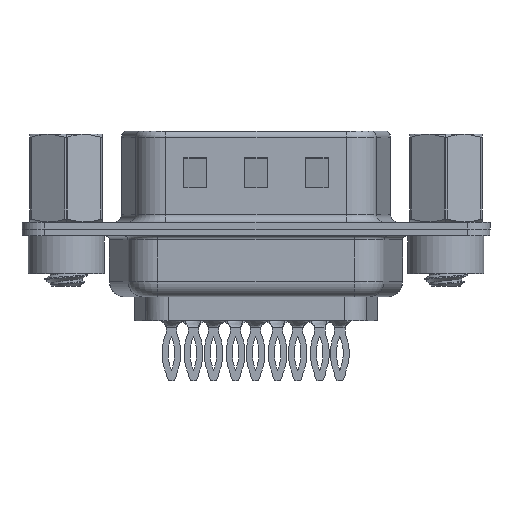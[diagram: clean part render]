
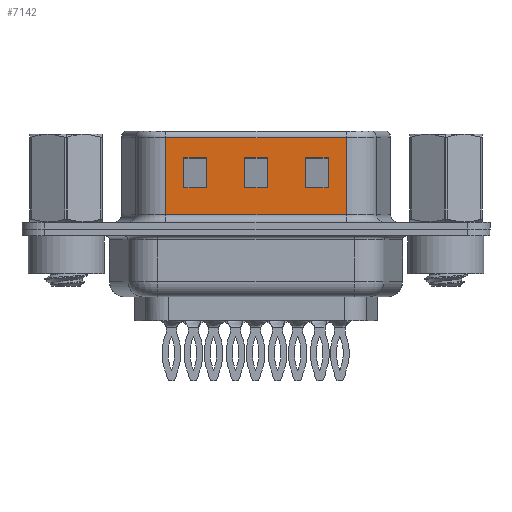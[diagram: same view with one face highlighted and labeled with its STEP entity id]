
A CAD part, front view. The second image highlights one B-rep face of the part: STEP entity #7142.
In plain terms, the highlighted planar face has unit normal (0, -1, 0).
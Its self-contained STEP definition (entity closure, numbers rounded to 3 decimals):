
#5 = CARTESIAN_POINT ( 'NONE',  ( 22.445, -4.58, 2.705 ) ) ;
#225 = LINE ( 'NONE', #5, #17846 ) ;
#281 = AXIS2_PLACEMENT_3D ( 'NONE', #5912, #15935, #12637 ) ;
#364 = LINE ( 'NONE', #13672, #9409 ) ;
#991 = VECTOR ( 'NONE', #17453, 1000. ) ;
#1026 = VECTOR ( 'NONE', #21370, 1000. ) ;
#1065 = VERTEX_POINT ( 'NONE', #5603 ) ;
#1172 = ORIENTED_EDGE ( 'NONE', *, *, #15927, .T. ) ;
#1427 = VECTOR ( 'NONE', #1695, 1000. ) ;
#1654 = CARTESIAN_POINT ( 'NONE',  ( 17.245, -4.58, 2.705 ) ) ;
#1695 = DIRECTION ( 'NONE',  ( 0., 0., -1. ) ) ;
#1793 = CARTESIAN_POINT ( 'NONE',  ( 18.445, -4.58, 6.02 ) ) ;
#1898 = DIRECTION ( 'NONE',  ( -1., 0., 0. ) ) ;
#2000 = CARTESIAN_POINT ( 'NONE',  ( 7.745, -4.58, 6.52 ) ) ;
#2476 = VERTEX_POINT ( 'NONE', #20648 ) ;
#2485 = LINE ( 'NONE', #5687, #7076 ) ;
#2727 = FACE_BOUND ( 'NONE', #14940, .T. ) ;
#2777 = LINE ( 'NONE', #15978, #19882 ) ;
#2922 = LINE ( 'NONE', #4166, #14982 ) ;
#3330 = EDGE_LOOP ( 'NONE', ( #14161, #1172, #11680, #15747 ) ) ;
#3653 = ORIENTED_EDGE ( 'NONE', *, *, #10242, .T. ) ;
#3658 = ORIENTED_EDGE ( 'NONE', *, *, #15259, .T. ) ;
#3674 = EDGE_CURVE ( 'NONE', #1065, #19030, #15326, .T. ) ;
#3750 = CARTESIAN_POINT ( 'NONE',  ( 18.445, -4.58, 0.95 ) ) ;
#3858 = EDGE_CURVE ( 'NONE', #8471, #17684, #20876, .T. ) ;
#4065 = VERTEX_POINT ( 'NONE', #12612 ) ;
#4166 = CARTESIAN_POINT ( 'NONE',  ( 18.445, -4.58, 6.52 ) ) ;
#4791 = CARTESIAN_POINT ( 'NONE',  ( 7.745, -4.58, 4.705 ) ) ;
#5521 = LINE ( 'NONE', #8393, #10117 ) ;
#5603 = CARTESIAN_POINT ( 'NONE',  ( 18.445, -4.58, 6.02 ) ) ;
#5687 = CARTESIAN_POINT ( 'NONE',  ( 9.245, -4.58, 6.52 ) ) ;
#5754 = CARTESIAN_POINT ( 'NONE',  ( 11.745, -4.58, 6.52 ) ) ;
#5912 = CARTESIAN_POINT ( 'NONE',  ( 18.445, -4.58, 6.52 ) ) ;
#5944 = ORIENTED_EDGE ( 'NONE', *, *, #3858, .T. ) ;
#6185 = CARTESIAN_POINT ( 'NONE',  ( 6.545, -4.58, 6.02 ) ) ;
#6193 = VERTEX_POINT ( 'NONE', #7801 ) ;
#6239 = FACE_OUTER_BOUND ( 'NONE', #19968, .T. ) ;
#6380 = VECTOR ( 'NONE', #11335, 1000. ) ;
#6663 = CARTESIAN_POINT ( 'NONE',  ( 17.245, -4.58, 4.705 ) ) ;
#6908 = EDGE_CURVE ( 'NONE', #2476, #15737, #14059, .T. ) ;
#7076 = VECTOR ( 'NONE', #19087, 1000. ) ;
#7142 = ADVANCED_FACE ( 'NONE', ( #17566, #2727, #9434, #6239 ), #11308, .F. ) ;
#7801 = CARTESIAN_POINT ( 'NONE',  ( 11.745, -4.58, 4.705 ) ) ;
#8067 = LINE ( 'NONE', #14779, #1026 ) ;
#8137 = ORIENTED_EDGE ( 'NONE', *, *, #3674, .T. ) ;
#8382 = LINE ( 'NONE', #10254, #10697 ) ;
#8393 = CARTESIAN_POINT ( 'NONE',  ( 15.745, -4.58, 6.52 ) ) ;
#8471 = VERTEX_POINT ( 'NONE', #14948 ) ;
#8583 = EDGE_CURVE ( 'NONE', #18231, #8471, #2485, .T. ) ;
#8639 = LINE ( 'NONE', #15351, #14020 ) ;
#8955 = VERTEX_POINT ( 'NONE', #4791 ) ;
#9123 = DIRECTION ( 'NONE',  ( 1., 0., 0. ) ) ;
#9203 = EDGE_LOOP ( 'NONE', ( #13097, #5944, #3658, #3653 ) ) ;
#9338 = ORIENTED_EDGE ( 'NONE', *, *, #15983, .T. ) ;
#9409 = VECTOR ( 'NONE', #16849, 1000. ) ;
#9434 = FACE_BOUND ( 'NONE', #3330, .T. ) ;
#9868 = ORIENTED_EDGE ( 'NONE', *, *, #12613, .T. ) ;
#9917 = VERTEX_POINT ( 'NONE', #21143 ) ;
#9960 = LINE ( 'NONE', #21500, #1427 ) ;
#10117 = VECTOR ( 'NONE', #18385, 1000. ) ;
#10242 = EDGE_CURVE ( 'NONE', #8955, #18231, #8382, .T. ) ;
#10254 = CARTESIAN_POINT ( 'NONE',  ( 14.445, -4.58, 4.705 ) ) ;
#10598 = LINE ( 'NONE', #2000, #15352 ) ;
#10697 = VECTOR ( 'NONE', #9123, 1000. ) ;
#11041 = CARTESIAN_POINT ( 'NONE',  ( 7.745, -4.58, 2.705 ) ) ;
#11055 = EDGE_CURVE ( 'NONE', #19030, #9917, #9960, .T. ) ;
#11245 = DIRECTION ( 'NONE',  ( 0., 0., -1. ) ) ;
#11308 = PLANE ( 'NONE',  #281 ) ;
#11335 = DIRECTION ( 'NONE',  ( -1., 0., 0. ) ) ;
#11680 = ORIENTED_EDGE ( 'NONE', *, *, #6908, .T. ) ;
#12158 = DIRECTION ( 'NONE',  ( 1., 0., 0. ) ) ;
#12289 = EDGE_CURVE ( 'NONE', #6193, #4065, #21260, .T. ) ;
#12291 = CARTESIAN_POINT ( 'NONE',  ( 15.745, -4.58, 2.705 ) ) ;
#12474 = DIRECTION ( 'NONE',  ( 0., 0., 1. ) ) ;
#12612 = CARTESIAN_POINT ( 'NONE',  ( 13.245, -4.58, 4.705 ) ) ;
#12613 = EDGE_CURVE ( 'NONE', #13253, #15501, #2777, .T. ) ;
#12637 = DIRECTION ( 'NONE',  ( 0., 0., 1. ) ) ;
#12755 = ORIENTED_EDGE ( 'NONE', *, *, #14931, .F. ) ;
#13097 = ORIENTED_EDGE ( 'NONE', *, *, #8583, .T. ) ;
#13253 = VERTEX_POINT ( 'NONE', #6663 ) ;
#13589 = VECTOR ( 'NONE', #16004, 1000. ) ;
#13672 = CARTESIAN_POINT ( 'NONE',  ( 13.245, -4.58, 6.52 ) ) ;
#14020 = VECTOR ( 'NONE', #12158, 1000. ) ;
#14059 = LINE ( 'NONE', #17239, #991 ) ;
#14118 = LINE ( 'NONE', #5754, #15498 ) ;
#14161 = ORIENTED_EDGE ( 'NONE', *, *, #12289, .T. ) ;
#14221 = DIRECTION ( 'NONE',  ( 0., 0., 1. ) ) ;
#14258 = VERTEX_POINT ( 'NONE', #3750 ) ;
#14417 = ORIENTED_EDGE ( 'NONE', *, *, #17082, .T. ) ;
#14779 = CARTESIAN_POINT ( 'NONE',  ( 22.445, -4.58, 4.705 ) ) ;
#14931 = EDGE_CURVE ( 'NONE', #1065, #14258, #2922, .T. ) ;
#14940 = EDGE_LOOP ( 'NONE', ( #9868, #21026, #9338, #17110 ) ) ;
#14948 = CARTESIAN_POINT ( 'NONE',  ( 9.245, -4.58, 2.705 ) ) ;
#14982 = VECTOR ( 'NONE', #21485, 1000. ) ;
#15259 = EDGE_CURVE ( 'NONE', #17684, #8955, #10598, .T. ) ;
#15326 = LINE ( 'NONE', #1793, #20735 ) ;
#15351 = CARTESIAN_POINT ( 'NONE',  ( 18.445, -4.58, 0.95 ) ) ;
#15352 = VECTOR ( 'NONE', #14221, 1000. ) ;
#15498 = VECTOR ( 'NONE', #12474, 1000. ) ;
#15501 = VERTEX_POINT ( 'NONE', #1654 ) ;
#15583 = ORIENTED_EDGE ( 'NONE', *, *, #11055, .T. ) ;
#15737 = VERTEX_POINT ( 'NONE', #17444 ) ;
#15747 = ORIENTED_EDGE ( 'NONE', *, *, #19170, .T. ) ;
#15892 = VERTEX_POINT ( 'NONE', #12291 ) ;
#15927 = EDGE_CURVE ( 'NONE', #4065, #2476, #364, .T. ) ;
#15935 = DIRECTION ( 'NONE',  ( 0., 1., 0. ) ) ;
#15978 = CARTESIAN_POINT ( 'NONE',  ( 17.245, -4.58, 6.52 ) ) ;
#15983 = EDGE_CURVE ( 'NONE', #15892, #17719, #5521, .T. ) ;
#16004 = DIRECTION ( 'NONE',  ( 1., 0., 0. ) ) ;
#16308 = EDGE_CURVE ( 'NONE', #15501, #15892, #225, .T. ) ;
#16821 = DIRECTION ( 'NONE',  ( -1., 0., 0. ) ) ;
#16849 = DIRECTION ( 'NONE',  ( 0., 0., -1. ) ) ;
#17082 = EDGE_CURVE ( 'NONE', #9917, #14258, #8639, .T. ) ;
#17110 = ORIENTED_EDGE ( 'NONE', *, *, #17312, .T. ) ;
#17239 = CARTESIAN_POINT ( 'NONE',  ( 18.445, -4.58, 2.705 ) ) ;
#17312 = EDGE_CURVE ( 'NONE', #17719, #13253, #8067, .T. ) ;
#17444 = CARTESIAN_POINT ( 'NONE',  ( 11.745, -4.58, 2.705 ) ) ;
#17453 = DIRECTION ( 'NONE',  ( -1., 0., 0. ) ) ;
#17566 = FACE_BOUND ( 'NONE', #9203, .T. ) ;
#17646 = CARTESIAN_POINT ( 'NONE',  ( 18.445, -4.58, 4.705 ) ) ;
#17684 = VERTEX_POINT ( 'NONE', #11041 ) ;
#17719 = VERTEX_POINT ( 'NONE', #17946 ) ;
#17846 = VECTOR ( 'NONE', #16821, 1000. ) ;
#17946 = CARTESIAN_POINT ( 'NONE',  ( 15.745, -4.58, 4.705 ) ) ;
#18119 = CARTESIAN_POINT ( 'NONE',  ( 9.245, -4.58, 4.705 ) ) ;
#18231 = VERTEX_POINT ( 'NONE', #18119 ) ;
#18385 = DIRECTION ( 'NONE',  ( 0., 0., 1. ) ) ;
#19030 = VERTEX_POINT ( 'NONE', #6185 ) ;
#19087 = DIRECTION ( 'NONE',  ( 0., 0., -1. ) ) ;
#19170 = EDGE_CURVE ( 'NONE', #15737, #6193, #14118, .T. ) ;
#19236 = CARTESIAN_POINT ( 'NONE',  ( 14.445, -4.58, 2.705 ) ) ;
#19882 = VECTOR ( 'NONE', #11245, 1000. ) ;
#19968 = EDGE_LOOP ( 'NONE', ( #12755, #8137, #15583, #14417 ) ) ;
#20648 = CARTESIAN_POINT ( 'NONE',  ( 13.245, -4.58, 2.705 ) ) ;
#20735 = VECTOR ( 'NONE', #1898, 1000. ) ;
#20876 = LINE ( 'NONE', #19236, #6380 ) ;
#21026 = ORIENTED_EDGE ( 'NONE', *, *, #16308, .T. ) ;
#21143 = CARTESIAN_POINT ( 'NONE',  ( 6.545, -4.58, 0.95 ) ) ;
#21260 = LINE ( 'NONE', #17646, #13589 ) ;
#21370 = DIRECTION ( 'NONE',  ( 1., 0., 0. ) ) ;
#21485 = DIRECTION ( 'NONE',  ( 0., 0., -1. ) ) ;
#21500 = CARTESIAN_POINT ( 'NONE',  ( 6.545, -4.58, 6.52 ) ) ;
